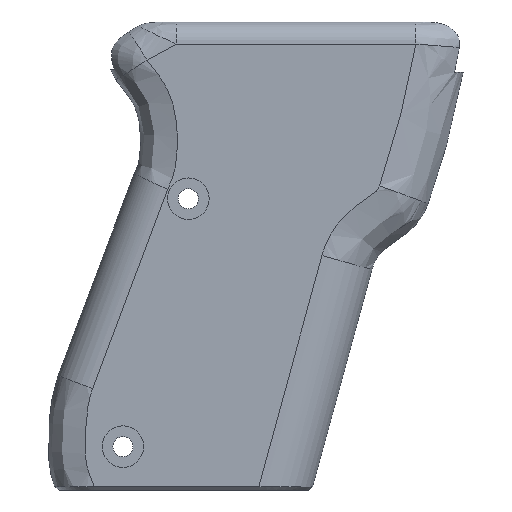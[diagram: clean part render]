
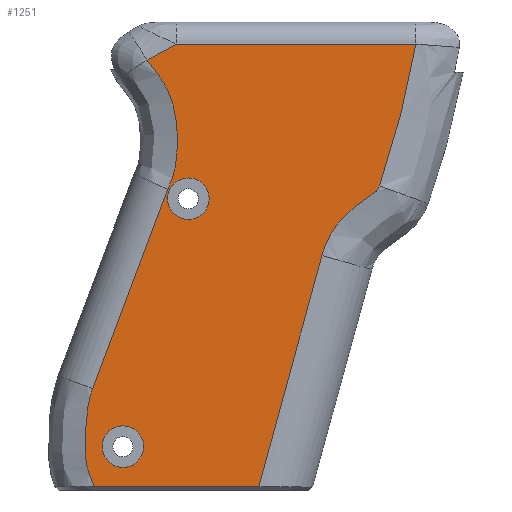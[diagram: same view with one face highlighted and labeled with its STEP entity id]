
A CAD part, front view. The second image highlights one B-rep face of the part: STEP entity #1251.
In plain terms, the highlighted planar face has unit normal (0, -1, 0).
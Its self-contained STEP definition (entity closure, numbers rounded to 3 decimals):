
#15=FACE_BOUND('',#401,.T.);
#16=FACE_BOUND('',#402,.T.);
#69=PLANE('',#1333);
#123=LINE('',#2323,#220);
#128=LINE('',#2602,#225);
#129=LINE('',#2629,#226);
#130=LINE('',#2650,#227);
#220=VECTOR('',#1473,10.);
#225=VECTOR('',#1482,8.);
#226=VECTOR('',#1483,10.);
#227=VECTOR('',#1484,10.);
#327=FACE_OUTER_BOUND('',#400,.T.);
#400=EDGE_LOOP('',(#963,#964,#965,#966,#967,#968,#969,#970,#971,#972,#973));
#401=EDGE_LOOP('',(#974));
#402=EDGE_LOOP('',(#975));
#459=CIRCLE('',#1334,3.1);
#460=CIRCLE('',#1335,3.1);
#505=B_SPLINE_CURVE_WITH_KNOTS('',3,(#2343,#2344,#2345,#2346),
 .UNSPECIFIED.,.F.,.F.,(4,4),(-0.899,-0.879),
 .UNSPECIFIED.);
#510=B_SPLINE_CURVE_WITH_KNOTS('',3,(#2409,#2410,#2411,#2412),
 .UNSPECIFIED.,.F.,.F.,(4,4),(-4.729,-4.712),
 .UNSPECIFIED.);
#513=B_SPLINE_CURVE_WITH_KNOTS('',3,(#2584,#2585,#2586,#2587,#2588,#2589,
#2590,#2591,#2592,#2593,#2594,#2595,#2596,#2597,#2598),.UNSPECIFIED.,.F.,
 .F.,(4,2,1,1,1,1,1,1,1,1,1,4),(-1.499,-1.331,-1.236,
-1.14,-1.045,-0.95,-0.76,
-0.57,-0.417,-0.38,-0.19,
0.),.UNSPECIFIED.);
#514=B_SPLINE_CURVE_WITH_KNOTS('',3,(#2604,#2605,#2606,#2607,#2608,#2609,
#2610,#2611,#2612,#2613,#2614,#2615,#2616,#2617,#2618,#2619,#2620),
 .UNSPECIFIED.,.F.,.F.,(4,1,1,1,1,1,1,1,1,1,1,1,1,1,4),(0.,
0.025,0.05,0.062,0.068,
0.074,0.087,0.099,0.124,
0.149,0.198,0.297,0.396,0.792,
1.387),.UNSPECIFIED.);
#515=B_SPLINE_CURVE_WITH_KNOTS('',3,(#2622,#2623,#2624,#2625,#2626,#2627),
 .UNSPECIFIED.,.F.,.F.,(4,1,1,4),(0.475,1.693,2.339,
2.661),.UNSPECIFIED.);
#516=B_SPLINE_CURVE_WITH_KNOTS('',3,(#2631,#2632,#2633,#2634,#2635,#2636),
 .UNSPECIFIED.,.F.,.F.,(4,2,4),(0.124,0.29,0.619),
 .UNSPECIFIED.);
#517=B_SPLINE_CURVE_WITH_KNOTS('',3,(#2638,#2639,#2640,#2641,#2642,#2643,
#2644,#2645,#2646,#2647,#2648,#2649),.UNSPECIFIED.,.F.,.F.,(4,1,1,1,1,1,
1,1,1,4),(-2.185,-1.944,-1.639,-1.334,
-1.029,-0.724,-0.419,-0.267,
-0.191,-0.114),.UNSPECIFIED.);
#574=VERTEX_POINT('',#2304);
#576=VERTEX_POINT('',#2320);
#577=VERTEX_POINT('',#2322);
#581=VERTEX_POINT('',#2380);
#585=VERTEX_POINT('',#2583);
#586=VERTEX_POINT('',#2601);
#587=VERTEX_POINT('',#2603);
#588=VERTEX_POINT('',#2621);
#589=VERTEX_POINT('',#2628);
#590=VERTEX_POINT('',#2630);
#591=VERTEX_POINT('',#2637);
#592=VERTEX_POINT('',#2651);
#593=VERTEX_POINT('',#2653);
#715=EDGE_CURVE('',#576,#577,#123,.T.);
#718=EDGE_CURVE('',#577,#574,#505,.T.);
#724=EDGE_CURVE('',#581,#576,#510,.T.);
#729=EDGE_CURVE('',#574,#585,#513,.T.);
#731=EDGE_CURVE('',#586,#581,#128,.T.);
#732=EDGE_CURVE('',#587,#586,#514,.T.);
#733=EDGE_CURVE('',#588,#587,#515,.T.);
#734=EDGE_CURVE('',#589,#588,#129,.T.);
#735=EDGE_CURVE('',#590,#589,#516,.T.);
#736=EDGE_CURVE('',#591,#590,#517,.T.);
#737=EDGE_CURVE('',#585,#591,#130,.T.);
#738=EDGE_CURVE('',#592,#592,#459,.T.);
#739=EDGE_CURVE('',#593,#593,#460,.T.);
#963=ORIENTED_EDGE('',*,*,#718,.F.);
#964=ORIENTED_EDGE('',*,*,#715,.F.);
#965=ORIENTED_EDGE('',*,*,#724,.F.);
#966=ORIENTED_EDGE('',*,*,#731,.F.);
#967=ORIENTED_EDGE('',*,*,#732,.F.);
#968=ORIENTED_EDGE('',*,*,#733,.F.);
#969=ORIENTED_EDGE('',*,*,#734,.F.);
#970=ORIENTED_EDGE('',*,*,#735,.F.);
#971=ORIENTED_EDGE('',*,*,#736,.F.);
#972=ORIENTED_EDGE('',*,*,#737,.F.);
#973=ORIENTED_EDGE('',*,*,#729,.F.);
#974=ORIENTED_EDGE('',*,*,#738,.T.);
#975=ORIENTED_EDGE('',*,*,#739,.T.);
#1251=ADVANCED_FACE('',(#327,#15,#16),#69,.F.);
#1333=AXIS2_PLACEMENT_3D('',#2600,#1480,#1481);
#1334=AXIS2_PLACEMENT_3D('',#2652,#1485,#1486);
#1335=AXIS2_PLACEMENT_3D('',#2654,#1487,#1488);
#1473=DIRECTION('',(-1.,0.,0.));
#1480=DIRECTION('center_axis',(0.,1.,0.));
#1481=DIRECTION('ref_axis',(1.,0.,0.));
#1482=DIRECTION('',(-0.264,0.,-0.965));
#1483=DIRECTION('',(1.,0.,0.));
#1484=DIRECTION('',(0.352,0.,0.936));
#1485=DIRECTION('center_axis',(0.,1.,0.));
#1486=DIRECTION('ref_axis',(1.,0.,0.));
#1487=DIRECTION('center_axis',(0.,1.,0.));
#1488=DIRECTION('ref_axis',(1.,0.,0.));
#2304=CARTESIAN_POINT('',(-11.469,-6.,-36.82));
#2320=CARTESIAN_POINT('',(12.972,-6.,-36.82));
#2322=CARTESIAN_POINT('',(-11.267,-6.,-36.82));
#2323=CARTESIAN_POINT('',(-1.923,-6.,-36.82));
#2343=CARTESIAN_POINT('Ctrl Pts',(-11.267,-6.,-36.82));
#2344=CARTESIAN_POINT('Ctrl Pts',(-11.335,-6.,-36.82));
#2345=CARTESIAN_POINT('Ctrl Pts',(-11.402,-6.,-36.82));
#2346=CARTESIAN_POINT('Ctrl Pts',(-11.469,-6.,-36.82));
#2380=CARTESIAN_POINT('',(13.109,-6.,-36.82));
#2409=CARTESIAN_POINT('Ctrl Pts',(13.109,-6.,-36.82));
#2410=CARTESIAN_POINT('Ctrl Pts',(13.063,-6.,-36.82));
#2411=CARTESIAN_POINT('Ctrl Pts',(13.018,-6.,-36.82));
#2412=CARTESIAN_POINT('Ctrl Pts',(12.972,-6.,-36.82));
#2583=CARTESIAN_POINT('',(-11.717,-6.,-22.176));
#2584=CARTESIAN_POINT('Ctrl Pts',(-11.469,-6.,-36.82));
#2585=CARTESIAN_POINT('Ctrl Pts',(-11.679,-6.,-36.301));
#2586=CARTESIAN_POINT('Ctrl Pts',(-11.888,-6.,-35.782));
#2587=CARTESIAN_POINT('Ctrl Pts',(-12.216,-6.,-34.968));
#2588=CARTESIAN_POINT('Ctrl Pts',(-12.429,-6.,-34.372));
#2589=CARTESIAN_POINT('Ctrl Pts',(-12.662,-6.,-33.448));
#2590=CARTESIAN_POINT('Ctrl Pts',(-12.79,-6.,-32.505));
#2591=CARTESIAN_POINT('Ctrl Pts',(-12.855,-6.,-31.238));
#2592=CARTESIAN_POINT('Ctrl Pts',(-12.838,-6.,-29.658));
#2593=CARTESIAN_POINT('Ctrl Pts',(-12.755,-6.,-27.887));
#2594=CARTESIAN_POINT('Ctrl Pts',(-12.645,-6.,-26.624));
#2595=CARTESIAN_POINT('Ctrl Pts',(-12.497,-6.,-25.366));
#2596=CARTESIAN_POINT('Ctrl Pts',(-12.28,-6.,-23.995));
#2597=CARTESIAN_POINT('Ctrl Pts',(-11.94,-6.,-22.769));
#2598=CARTESIAN_POINT('Ctrl Pts',(-11.717,-6.,-22.176));
#2600=CARTESIAN_POINT('Origin',(13.353,-6.,-2.363));
#2601=CARTESIAN_POINT('',(22.536,-6.,-2.313));
#2602=CARTESIAN_POINT('',(13.53,-6.,-35.279));
#2603=CARTESIAN_POINT('',(31.135,-6.,8.136));
#2604=CARTESIAN_POINT('Ctrl Pts',(31.135,-6.,8.136));
#2605=CARTESIAN_POINT('Ctrl Pts',(31.106,-6.,8.058));
#2606=CARTESIAN_POINT('Ctrl Pts',(31.046,-6.,7.905));
#2607=CARTESIAN_POINT('Ctrl Pts',(30.957,-6.,7.718));
#2608=CARTESIAN_POINT('Ctrl Pts',(30.884,-6.,7.593));
#2609=CARTESIAN_POINT('Ctrl Pts',(30.837,-6.,7.525));
#2610=CARTESIAN_POINT('Ctrl Pts',(30.786,-6.,7.46));
#2611=CARTESIAN_POINT('Ctrl Pts',(30.714,-6.,7.385));
#2612=CARTESIAN_POINT('Ctrl Pts',(30.593,-6.,7.274));
#2613=CARTESIAN_POINT('Ctrl Pts',(30.432,-6.,7.143));
#2614=CARTESIAN_POINT('Ctrl Pts',(30.168,-6.,6.944));
#2615=CARTESIAN_POINT('Ctrl Pts',(29.695,-6.,6.614));
#2616=CARTESIAN_POINT('Ctrl Pts',(29.008,-6.,6.154));
#2617=CARTESIAN_POINT('Ctrl Pts',(27.382,-6.,5.027));
#2618=CARTESIAN_POINT('Ctrl Pts',(24.614,-6.,2.614));
#2619=CARTESIAN_POINT('Ctrl Pts',(23.058,-6.,-0.401));
#2620=CARTESIAN_POINT('Ctrl Pts',(22.536,-6.,-2.313));
#2621=CARTESIAN_POINT('',(36.563,-6.,29.294));
#2622=CARTESIAN_POINT('Ctrl Pts',(36.563,-6.,29.294));
#2623=CARTESIAN_POINT('Ctrl Pts',(35.796,-6.,25.306));
#2624=CARTESIAN_POINT('Ctrl Pts',(34.531,-6.,19.22));
#2625=CARTESIAN_POINT('Ctrl Pts',(32.566,-6.,12.195));
#2626=CARTESIAN_POINT('Ctrl Pts',(31.508,-6.,9.145));
#2627=CARTESIAN_POINT('Ctrl Pts',(31.135,-6.,8.136));
#2628=CARTESIAN_POINT('',(0.757,-6.,29.294));
#2629=CARTESIAN_POINT('',(29.204,-6.,29.294));
#2630=CARTESIAN_POINT('',(-3.579,-6.,26.911));
#2631=CARTESIAN_POINT('Ctrl Pts',(-3.579,-6.,26.911));
#2632=CARTESIAN_POINT('Ctrl Pts',(-3.111,-6.,27.209));
#2633=CARTESIAN_POINT('Ctrl Pts',(-2.626,-6.,27.484));
#2634=CARTESIAN_POINT('Ctrl Pts',(-1.172,-6.,28.262));
#2635=CARTESIAN_POINT('Ctrl Pts',(-0.207,-6.,
28.778));
#2636=CARTESIAN_POINT('Ctrl Pts',(0.757,-6.,29.294));
#2637=CARTESIAN_POINT('',(-0.516,-6.,7.589));
#2638=CARTESIAN_POINT('Ctrl Pts',(-0.516,-6.,
7.589));
#2639=CARTESIAN_POINT('Ctrl Pts',(-0.139,-6.,
8.298));
#2640=CARTESIAN_POINT('Ctrl Pts',(0.525,-6.,10.006));
#2641=CARTESIAN_POINT('Ctrl Pts',(0.933,-6.,12.824));
#2642=CARTESIAN_POINT('Ctrl Pts',(0.979,-6.,15.873));
#2643=CARTESIAN_POINT('Ctrl Pts',(0.701,-6.,18.917));
#2644=CARTESIAN_POINT('Ctrl Pts',(-0.142,-6.,21.868));
#2645=CARTESIAN_POINT('Ctrl Pts',(-1.409,-6.,24.094));
#2646=CARTESIAN_POINT('Ctrl Pts',(-2.503,-6.,25.497));
#2647=CARTESIAN_POINT('Ctrl Pts',(-3.139,-6.,26.289));
#2648=CARTESIAN_POINT('Ctrl Pts',(-3.443,-6.,26.697));
#2649=CARTESIAN_POINT('Ctrl Pts',(-3.579,-6.,26.911));
#2650=CARTESIAN_POINT('',(-1.221,-6.,5.715));
#2651=CARTESIAN_POINT('',(-0.516,-6.,6.198));
#2652=CARTESIAN_POINT('Origin',(2.584,-6.,6.198));
#2653=CARTESIAN_POINT('',(-10.292,-6.,-30.834));
#2654=CARTESIAN_POINT('Origin',(-7.192,-6.,-30.834));
